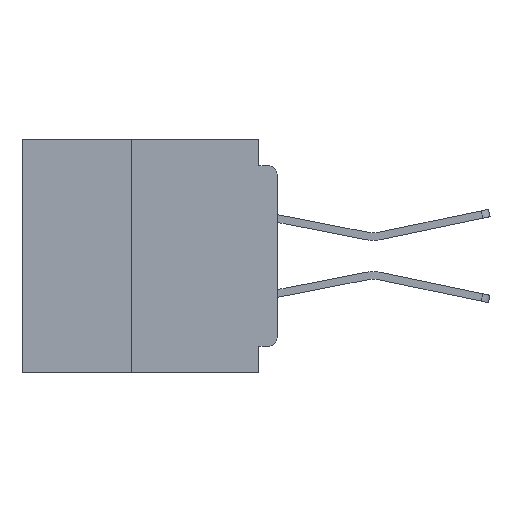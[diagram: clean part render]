
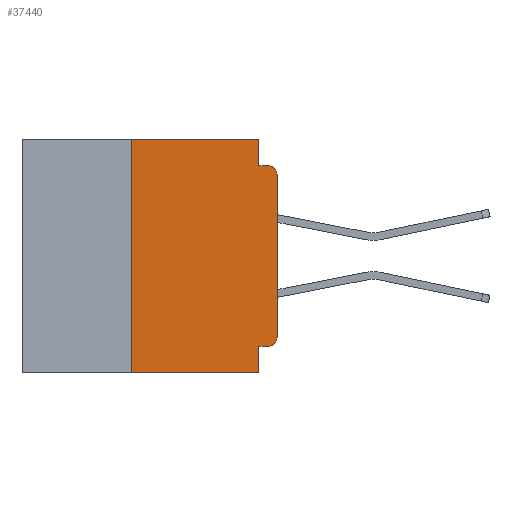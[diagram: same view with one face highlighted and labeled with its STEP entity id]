
A CAD part, left-side view. The second image highlights one B-rep face of the part: STEP entity #37440.
In plain terms, the highlighted planar face has unit normal (-1, 0, 0).
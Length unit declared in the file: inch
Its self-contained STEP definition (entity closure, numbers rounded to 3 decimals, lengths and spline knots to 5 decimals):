
#568 = EDGE_LOOP ( 'NONE', ( #3949, #7241, #52403, #16408, #18287, #25207, #6113, #20187, #10388, #2006 ) ) ;
#571 = CARTESIAN_POINT ( 'NONE',  ( 0., 0.015, -0.34 ) ) ;
#1135 = VERTEX_POINT ( 'NONE', #17996 ) ;
#1753 = VERTEX_POINT ( 'NONE', #31348 ) ;
#2006 = ORIENTED_EDGE ( 'NONE', *, *, #17176, .T. ) ;
#2786 = DIRECTION ( 'NONE',  ( 0., 0., 1. ) ) ;
#2891 = DIRECTION ( 'NONE',  ( 1., 0., 0. ) ) ;
#3949 = ORIENTED_EDGE ( 'NONE', *, *, #40576, .T. ) ;
#4407 = CIRCLE ( 'NONE', #9669, 0.015 ) ;
#4476 = LINE ( 'NONE', #8124, #48595 ) ;
#4720 = CARTESIAN_POINT ( 'NONE',  ( 0., 0., 0. ) ) ;
#4908 = VERTEX_POINT ( 'NONE', #17266 ) ;
#4932 = DIRECTION ( 'NONE',  ( 0., 0., -1. ) ) ;
#5631 = VECTOR ( 'NONE', #10661, 39.37008 ) ;
#6113 = ORIENTED_EDGE ( 'NONE', *, *, #34057, .T. ) ;
#7241 = ORIENTED_EDGE ( 'NONE', *, *, #9348, .T. ) ;
#8124 = CARTESIAN_POINT ( 'NONE',  ( 0., 0., -0.045 ) ) ;
#8245 = VECTOR ( 'NONE', #15610, 39.37008 ) ;
#8838 = VECTOR ( 'NONE', #2786, 39.37008 ) ;
#8960 = VERTEX_POINT ( 'NONE', #20779 ) ;
#9348 = EDGE_CURVE ( 'NONE', #40733, #20235, #4407, .T. ) ;
#9669 = AXIS2_PLACEMENT_3D ( 'NONE', #36012, #10487, #40294 ) ;
#9728 = VECTOR ( 'NONE', #51770, 39.37008 ) ;
#10028 = CARTESIAN_POINT ( 'NONE',  ( 0., 0., -0.06 ) ) ;
#10388 = ORIENTED_EDGE ( 'NONE', *, *, #49115, .F. ) ;
#10487 = DIRECTION ( 'NONE',  ( -1., 0., 0. ) ) ;
#10661 = DIRECTION ( 'NONE',  ( 0., -1., 0. ) ) ;
#10865 = LINE ( 'NONE', #50463, #12206 ) ;
#10880 = AXIS2_PLACEMENT_3D ( 'NONE', #571, #30595, #4932 ) ;
#12206 = VECTOR ( 'NONE', #20670, 39.37008 ) ;
#13578 = VECTOR ( 'NONE', #23076, 39.37008 ) ;
#14090 = DIRECTION ( 'NONE',  ( 0., 0., -1. ) ) ;
#15610 = DIRECTION ( 'NONE',  ( 0., 0., -1. ) ) ;
#15754 = PLANE ( 'NONE',  #44751 ) ;
#16408 = ORIENTED_EDGE ( 'NONE', *, *, #35270, .F. ) ;
#17149 = VERTEX_POINT ( 'NONE', #34697 ) ;
#17176 = EDGE_CURVE ( 'NONE', #1753, #43332, #35275, .T. ) ;
#17247 = CARTESIAN_POINT ( 'NONE',  ( 0., 0., -0.34 ) ) ;
#17266 = CARTESIAN_POINT ( 'NONE',  ( 0., 0.031, 0. ) ) ;
#17665 = CARTESIAN_POINT ( 'NONE',  ( 0., 0.015, -0.045 ) ) ;
#17996 = CARTESIAN_POINT ( 'NONE',  ( 0., 0.25, -0.4 ) ) ;
#18287 = ORIENTED_EDGE ( 'NONE', *, *, #42301, .F. ) ;
#19633 = LINE ( 'NONE', #28250, #8245 ) ;
#20187 = ORIENTED_EDGE ( 'NONE', *, *, #29894, .F. ) ;
#20235 = VERTEX_POINT ( 'NONE', #17665 ) ;
#20670 = DIRECTION ( 'NONE',  ( 0., 1., 0. ) ) ;
#20779 = CARTESIAN_POINT ( 'NONE',  ( 0., 0.031, -0.4 ) ) ;
#23076 = DIRECTION ( 'NONE',  ( 0., -1., 0. ) ) ;
#23922 = VERTEX_POINT ( 'NONE', #27014 ) ;
#24265 = CARTESIAN_POINT ( 'NONE',  ( 0., 0.437, 0. ) ) ;
#25207 = ORIENTED_EDGE ( 'NONE', *, *, #26765, .F. ) ;
#26765 = EDGE_CURVE ( 'NONE', #1135, #23922, #30209, .T. ) ;
#27014 = CARTESIAN_POINT ( 'NONE',  ( 0., 0.25, 0. ) ) ;
#27365 = CARTESIAN_POINT ( 'NONE',  ( 0., 0.437, 0. ) ) ;
#28250 = CARTESIAN_POINT ( 'NONE',  ( 0., 0.031, 0. ) ) ;
#29668 = EDGE_CURVE ( 'NONE', #17149, #20235, #4476, .T. ) ;
#29894 = EDGE_CURVE ( 'NONE', #33080, #8960, #49229, .T. ) ;
#30209 = LINE ( 'NONE', #45592, #8838 ) ;
#30595 = DIRECTION ( 'NONE',  ( -1., 0., 0. ) ) ;
#31348 = CARTESIAN_POINT ( 'NONE',  ( 0., 0.015, -0.355 ) ) ;
#31904 = CARTESIAN_POINT ( 'NONE',  ( 0., 0.437, -0.4 ) ) ;
#32851 = DIRECTION ( 'NONE',  ( 0., 0., -1. ) ) ;
#33080 = VERTEX_POINT ( 'NONE', #50905 ) ;
#34057 = EDGE_CURVE ( 'NONE', #1135, #8960, #51067, .T. ) ;
#34697 = CARTESIAN_POINT ( 'NONE',  ( 0., 0.031, -0.045 ) ) ;
#35270 = EDGE_CURVE ( 'NONE', #4908, #17149, #19633, .T. ) ;
#35275 = CIRCLE ( 'NONE', #10880, 0.015 ) ;
#36012 = CARTESIAN_POINT ( 'NONE',  ( 0., 0.015, -0.06 ) ) ;
#37440 = ADVANCED_FACE ( 'NONE', ( #40802 ), #15754, .F. ) ;
#37901 = VECTOR ( 'NONE', #14090, 39.37008 ) ;
#39599 = CARTESIAN_POINT ( 'NONE',  ( 0., 0.031, -0.4 ) ) ;
#40294 = DIRECTION ( 'NONE',  ( 0., 0., -1. ) ) ;
#40576 = EDGE_CURVE ( 'NONE', #43332, #40733, #55047, .T. ) ;
#40733 = VERTEX_POINT ( 'NONE', #10028 ) ;
#40802 = FACE_OUTER_BOUND ( 'NONE', #568, .T. ) ;
#42250 = DIRECTION ( 'NONE',  ( 0., -1., 0. ) ) ;
#42301 = EDGE_CURVE ( 'NONE', #23922, #4908, #47553, .T. ) ;
#43332 = VERTEX_POINT ( 'NONE', #17247 ) ;
#44751 = AXIS2_PLACEMENT_3D ( 'NONE', #24265, #2891, #32851 ) ;
#45592 = CARTESIAN_POINT ( 'NONE',  ( 0., 0.25, -0.4 ) ) ;
#47553 = LINE ( 'NONE', #27365, #13578 ) ;
#48595 = VECTOR ( 'NONE', #42250, 39.37008 ) ;
#49115 = EDGE_CURVE ( 'NONE', #1753, #33080, #10865, .T. ) ;
#49229 = LINE ( 'NONE', #39599, #37901 ) ;
#50463 = CARTESIAN_POINT ( 'NONE',  ( 0., 0., -0.355 ) ) ;
#50905 = CARTESIAN_POINT ( 'NONE',  ( 0., 0.031, -0.355 ) ) ;
#51067 = LINE ( 'NONE', #31904, #5631 ) ;
#51770 = DIRECTION ( 'NONE',  ( 0., 0., 1. ) ) ;
#52403 = ORIENTED_EDGE ( 'NONE', *, *, #29668, .F. ) ;
#55047 = LINE ( 'NONE', #4720, #9728 ) ;
